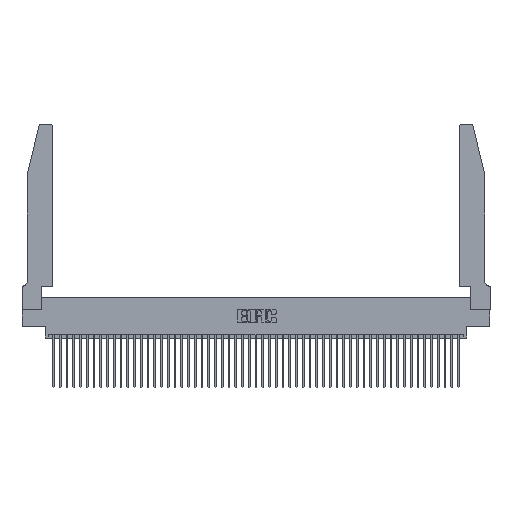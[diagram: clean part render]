
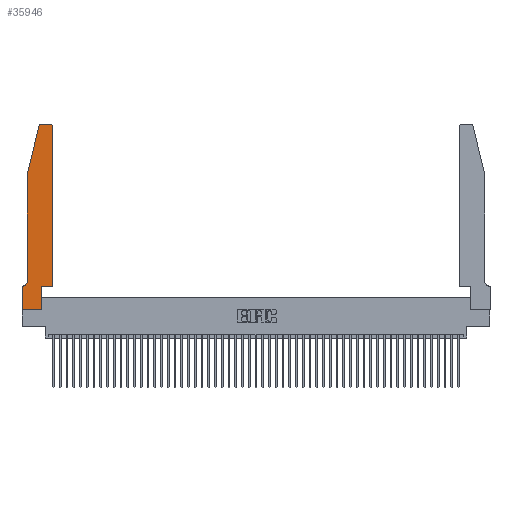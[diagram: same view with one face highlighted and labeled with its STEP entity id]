
A CAD part, top view. The second image highlights one B-rep face of the part: STEP entity #35946.
In plain terms, the highlighted planar face has unit normal (0, 0, 1).
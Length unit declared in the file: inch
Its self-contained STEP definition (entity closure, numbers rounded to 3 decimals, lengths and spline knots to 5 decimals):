
#971 = DIRECTION ( 'NONE',  ( 0., -1., 0. ) ) ;
#1722 = DIRECTION ( 'NONE',  ( -1., 0., 0. ) ) ;
#1891 = LINE ( 'NONE', #1946, #45570 ) ;
#1946 = CARTESIAN_POINT ( 'NONE',  ( 0.2865, 0.35, 0.37 ) ) ;
#2374 = ORIENTED_EDGE ( 'NONE', *, *, #39576, .T. ) ;
#2782 = DIRECTION ( 'NONE',  ( 0., 0., 1. ) ) ;
#2884 = DIRECTION ( 'NONE',  ( -1., 0., 0. ) ) ;
#3454 = ORIENTED_EDGE ( 'NONE', *, *, #23350, .T. ) ;
#4196 = VERTEX_POINT ( 'NONE', #33515 ) ;
#4438 = VERTEX_POINT ( 'NONE', #12035 ) ;
#6500 = VERTEX_POINT ( 'NONE', #6854 ) ;
#6854 = CARTESIAN_POINT ( 'NONE',  ( 0.0755, 0.42, 0.37 ) ) ;
#7072 = EDGE_CURVE ( 'NONE', #22373, #49301, #48616, .T. ) ;
#7886 = DIRECTION ( 'NONE',  ( 0., -1., 0. ) ) ;
#8004 = VECTOR ( 'NONE', #971, 39.37008 ) ;
#8992 = EDGE_LOOP ( 'NONE', ( #27709, #42197, #48416, #2374, #16023, #17041, #45076, #13788, #11292, #25231, #3454, #24138 ) ) ;
#10015 = DIRECTION ( 'NONE',  ( 1., 0., 0. ) ) ;
#10046 = VERTEX_POINT ( 'NONE', #24538 ) ;
#10864 = CARTESIAN_POINT ( 'NONE',  ( 0.2605, 2.75, 0.37 ) ) ;
#11292 = ORIENTED_EDGE ( 'NONE', *, *, #38885, .T. ) ;
#11518 = VERTEX_POINT ( 'NONE', #33510 ) ;
#12035 = CARTESIAN_POINT ( 'NONE',  ( 0.0755, 2., 0.37 ) ) ;
#12460 = CARTESIAN_POINT ( 'NONE',  ( 0., 0., 0.37 ) ) ;
#13395 = FACE_OUTER_BOUND ( 'NONE', #8992, .T. ) ;
#13788 = ORIENTED_EDGE ( 'NONE', *, *, #30490, .T. ) ;
#15257 = CIRCLE ( 'NONE', #46196, 0.03 ) ;
#16023 = ORIENTED_EDGE ( 'NONE', *, *, #30526, .T. ) ;
#16178 = VECTOR ( 'NONE', #2884, 39.37008 ) ;
#16673 = LINE ( 'NONE', #48154, #35963 ) ;
#17041 = ORIENTED_EDGE ( 'NONE', *, *, #44388, .T. ) ;
#17089 = CARTESIAN_POINT ( 'NONE',  ( 0.4505, 0.35, 0.37 ) ) ;
#17503 = LINE ( 'NONE', #33285, #46927 ) ;
#18492 = CARTESIAN_POINT ( 'NONE',  ( 0.0055, 0.42, 0.37 ) ) ;
#19288 = EDGE_CURVE ( 'NONE', #10046, #11518, #15257, .T. ) ;
#20131 = VERTEX_POINT ( 'NONE', #45740 ) ;
#21503 = CARTESIAN_POINT ( 'NONE',  ( 0.284, 2.72, 0.37 ) ) ;
#22355 = DIRECTION ( 'NONE',  ( -1., 0., 0. ) ) ;
#22373 = VERTEX_POINT ( 'NONE', #49030 ) ;
#23350 = EDGE_CURVE ( 'NONE', #29550, #22373, #32299, .T. ) ;
#24014 = LINE ( 'NONE', #10864, #16178 ) ;
#24138 = ORIENTED_EDGE ( 'NONE', *, *, #7072, .T. ) ;
#24538 = CARTESIAN_POINT ( 'NONE',  ( 0.284, 2.75, 0.37 ) ) ;
#24817 = DIRECTION ( 'NONE',  ( 0., 1., 0. ) ) ;
#25231 = ORIENTED_EDGE ( 'NONE', *, *, #41054, .T. ) ;
#25343 = DIRECTION ( 'NONE',  ( 1., 0., 0. ) ) ;
#25344 = VECTOR ( 'NONE', #7886, 39.37008 ) ;
#26170 = CARTESIAN_POINT ( 'NONE',  ( 0.4205, 2.72, 0.37 ) ) ;
#27709 = ORIENTED_EDGE ( 'NONE', *, *, #47441, .T. ) ;
#27838 = VECTOR ( 'NONE', #29704, 39.37008 ) ;
#28195 = AXIS2_PLACEMENT_3D ( 'NONE', #18492, #45310, #22355 ) ;
#28341 = VERTEX_POINT ( 'NONE', #45497 ) ;
#28373 = VERTEX_POINT ( 'NONE', #34308 ) ;
#28689 = LINE ( 'NONE', #47437, #8004 ) ;
#29053 = LINE ( 'NONE', #37466, #27838 ) ;
#29256 = DIRECTION ( 'NONE',  ( 0., 1., 0. ) ) ;
#29550 = VERTEX_POINT ( 'NONE', #37734 ) ;
#29704 = DIRECTION ( 'NONE',  ( 1., 0., 0. ) ) ;
#30073 = DIRECTION ( 'NONE',  ( 1., 0., 0. ) ) ;
#30437 = AXIS2_PLACEMENT_3D ( 'NONE', #26170, #2782, #30073 ) ;
#30490 = EDGE_CURVE ( 'NONE', #49004, #28373, #17503, .T. ) ;
#30526 = EDGE_CURVE ( 'NONE', #6500, #28341, #33138, .T. ) ;
#31079 = VECTOR ( 'NONE', #24817, 39.37008 ) ;
#32299 = LINE ( 'NONE', #17089, #31079 ) ;
#33138 = CIRCLE ( 'NONE', #28195, 0.07 ) ;
#33214 = DIRECTION ( 'NONE',  ( 0., 0., 1. ) ) ;
#33285 = CARTESIAN_POINT ( 'NONE',  ( 0., 0., 0.37 ) ) ;
#33510 = CARTESIAN_POINT ( 'NONE',  ( 0.25487, 2.72718, 0.37 ) ) ;
#33515 = CARTESIAN_POINT ( 'NONE',  ( 0., 0.35, 0.37 ) ) ;
#34308 = CARTESIAN_POINT ( 'NONE',  ( 0.2865, 0., 0.37 ) ) ;
#34922 = CARTESIAN_POINT ( 'NONE',  ( 0.0755, 2., 0.37 ) ) ;
#35946 = ADVANCED_FACE ( 'NONE', ( #13395 ), #40587, .T. ) ;
#35963 = VECTOR ( 'NONE', #1722, 39.37008 ) ;
#36288 = LINE ( 'NONE', #34922, #45219 ) ;
#37398 = CARTESIAN_POINT ( 'NONE',  ( 0.4205, 2.75, 0.37 ) ) ;
#37466 = CARTESIAN_POINT ( 'NONE',  ( 0.4505, 0.35, 0.37 ) ) ;
#37734 = CARTESIAN_POINT ( 'NONE',  ( 0.4505, 0.35, 0.37 ) ) ;
#38885 = EDGE_CURVE ( 'NONE', #28373, #20131, #1891, .T. ) ;
#39576 = EDGE_CURVE ( 'NONE', #4438, #6500, #28689, .T. ) ;
#40587 = PLANE ( 'NONE',  #45672 ) ;
#40745 = CARTESIAN_POINT ( 'NONE',  ( 0., 0.35, 0.37 ) ) ;
#41054 = EDGE_CURVE ( 'NONE', #20131, #29550, #29053, .T. ) ;
#41284 = EDGE_CURVE ( 'NONE', #11518, #4438, #36288, .T. ) ;
#41958 = EDGE_CURVE ( 'NONE', #4196, #49004, #45747, .T. ) ;
#42197 = ORIENTED_EDGE ( 'NONE', *, *, #19288, .T. ) ;
#42610 = DIRECTION ( 'NONE',  ( -0.239, -0.971, 0. ) ) ;
#43219 = CARTESIAN_POINT ( 'NONE',  ( 0., 0., 0.37 ) ) ;
#44388 = EDGE_CURVE ( 'NONE', #28341, #4196, #16673, .T. ) ;
#44820 = DIRECTION ( 'NONE',  ( 1., 0., 0. ) ) ;
#45076 = ORIENTED_EDGE ( 'NONE', *, *, #41958, .T. ) ;
#45219 = VECTOR ( 'NONE', #42610, 39.37008 ) ;
#45310 = DIRECTION ( 'NONE',  ( 0., 0., -1. ) ) ;
#45497 = CARTESIAN_POINT ( 'NONE',  ( 0.0055, 0.35, 0.37 ) ) ;
#45570 = VECTOR ( 'NONE', #29256, 39.37008 ) ;
#45672 = AXIS2_PLACEMENT_3D ( 'NONE', #40745, #33214, #10015 ) ;
#45740 = CARTESIAN_POINT ( 'NONE',  ( 0.2865, 0.35, 0.37 ) ) ;
#45747 = LINE ( 'NONE', #43219, #25344 ) ;
#46196 = AXIS2_PLACEMENT_3D ( 'NONE', #21503, #48332, #25343 ) ;
#46927 = VECTOR ( 'NONE', #44820, 39.37008 ) ;
#47437 = CARTESIAN_POINT ( 'NONE',  ( 0.0755, 2., 0.37 ) ) ;
#47441 = EDGE_CURVE ( 'NONE', #49301, #10046, #24014, .T. ) ;
#48154 = CARTESIAN_POINT ( 'NONE',  ( 0.0755, 0.35, 0.37 ) ) ;
#48332 = DIRECTION ( 'NONE',  ( 0., 0., 1. ) ) ;
#48416 = ORIENTED_EDGE ( 'NONE', *, *, #41284, .T. ) ;
#48616 = CIRCLE ( 'NONE', #30437, 0.03 ) ;
#49004 = VERTEX_POINT ( 'NONE', #12460 ) ;
#49030 = CARTESIAN_POINT ( 'NONE',  ( 0.4505, 2.72, 0.37 ) ) ;
#49301 = VERTEX_POINT ( 'NONE', #37398 ) ;
